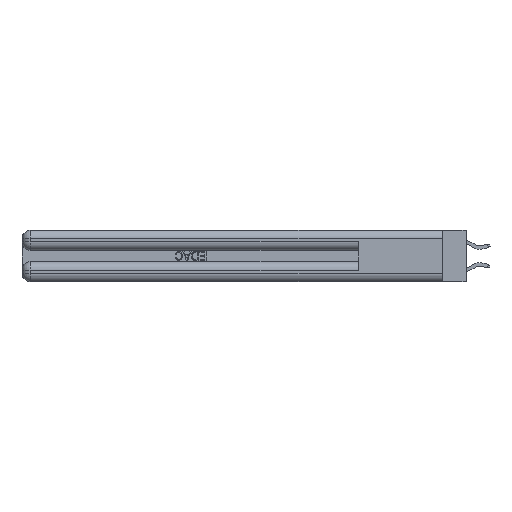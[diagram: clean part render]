
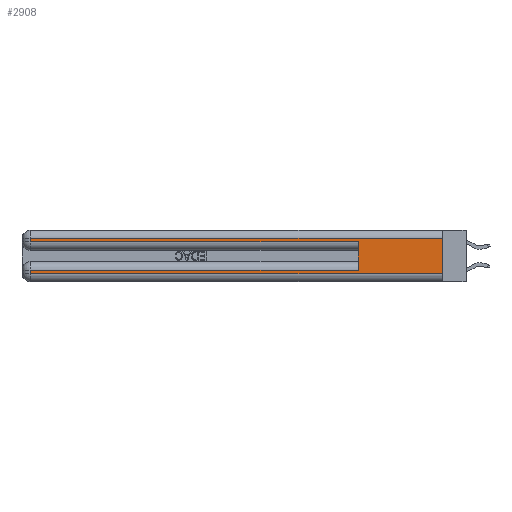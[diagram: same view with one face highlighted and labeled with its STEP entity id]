
A CAD part, left-side view. The second image highlights one B-rep face of the part: STEP entity #2908.
In plain terms, the highlighted planar face has unit normal (-1, 0, 0).
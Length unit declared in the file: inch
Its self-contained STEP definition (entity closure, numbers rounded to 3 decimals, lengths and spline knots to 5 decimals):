
#225 = ORIENTED_EDGE ( 'NONE', *, *, #33813, .T. ) ;
#605 = VERTEX_POINT ( 'NONE', #23759 ) ;
#2132 = EDGE_CURVE ( 'NONE', #27821, #29913, #11934, .T. ) ;
#2157 = VECTOR ( 'NONE', #27868, 39.37008 ) ;
#2297 = VERTEX_POINT ( 'NONE', #30778 ) ;
#2908 = ADVANCED_FACE ( 'NONE', ( #24517 ), #19023, .F. ) ;
#3054 = CARTESIAN_POINT ( 'NONE',  ( 0., 0., 0.37 ) ) ;
#3817 = VERTEX_POINT ( 'NONE', #20271 ) ;
#4042 = VECTOR ( 'NONE', #32883, 39.37008 ) ;
#4208 = EDGE_CURVE ( 'NONE', #2297, #29913, #4775, .T. ) ;
#4294 = LINE ( 'NONE', #22469, #11377 ) ;
#4775 = LINE ( 'NONE', #24913, #25253 ) ;
#4833 = CARTESIAN_POINT ( 'NONE',  ( 0., 2.94, 0.37 ) ) ;
#5351 = DIRECTION ( 'NONE',  ( 0., -1., 0. ) ) ;
#5700 = DIRECTION ( 'NONE',  ( 0., 0., -1. ) ) ;
#5804 = LINE ( 'NONE', #32035, #13721 ) ;
#6391 = CARTESIAN_POINT ( 'NONE',  ( 0., 2.94, 0.285 ) ) ;
#6636 = VERTEX_POINT ( 'NONE', #18787 ) ;
#6854 = CARTESIAN_POINT ( 'NONE',  ( 0., 2.94, 0.085 ) ) ;
#7870 = VECTOR ( 'NONE', #5351, 39.37008 ) ;
#8067 = ORIENTED_EDGE ( 'NONE', *, *, #21373, .T. ) ;
#8251 = CARTESIAN_POINT ( 'NONE',  ( 0., 2.94, 0.37 ) ) ;
#8323 = ORIENTED_EDGE ( 'NONE', *, *, #4208, .F. ) ;
#8755 = ORIENTED_EDGE ( 'NONE', *, *, #17038, .T. ) ;
#9690 = ORIENTED_EDGE ( 'NONE', *, *, #26692, .T. ) ;
#10274 = VERTEX_POINT ( 'NONE', #22075 ) ;
#10942 = DIRECTION ( 'NONE',  ( 0., 0., -1. ) ) ;
#11377 = VECTOR ( 'NONE', #33187, 39.37008 ) ;
#11934 = LINE ( 'NONE', #16774, #4042 ) ;
#13270 = CARTESIAN_POINT ( 'NONE',  ( 0., 0., 0.06 ) ) ;
#13721 = VECTOR ( 'NONE', #24103, 39.37008 ) ;
#14978 = LINE ( 'NONE', #13270, #7870 ) ;
#15521 = ORIENTED_EDGE ( 'NONE', *, *, #23359, .F. ) ;
#16385 = DIRECTION ( 'NONE',  ( 0., 0., 1. ) ) ;
#16407 = LINE ( 'NONE', #4833, #29780 ) ;
#16774 = CARTESIAN_POINT ( 'NONE',  ( 0., 0., 0.285 ) ) ;
#17038 = EDGE_CURVE ( 'NONE', #6636, #3817, #14978, .T. ) ;
#18787 = CARTESIAN_POINT ( 'NONE',  ( 0., 2.94, 0.06 ) ) ;
#19023 = PLANE ( 'NONE',  #24604 ) ;
#19372 = CARTESIAN_POINT ( 'NONE',  ( 0., 0.6, 0.285 ) ) ;
#20271 = CARTESIAN_POINT ( 'NONE',  ( 0., 0., 0.06 ) ) ;
#21373 = EDGE_CURVE ( 'NONE', #605, #27821, #16407, .T. ) ;
#21737 = DIRECTION ( 'NONE',  ( 1., 0., 0. ) ) ;
#22075 = CARTESIAN_POINT ( 'NONE',  ( 0., 0., 0.31 ) ) ;
#22469 = CARTESIAN_POINT ( 'NONE',  ( 0., 0., 0.085 ) ) ;
#23115 = EDGE_LOOP ( 'NONE', ( #15521, #25544, #8067, #25269, #8323, #9690, #225, #8755 ) ) ;
#23359 = EDGE_CURVE ( 'NONE', #10274, #3817, #5804, .T. ) ;
#23451 = LINE ( 'NONE', #25200, #2157 ) ;
#23759 = CARTESIAN_POINT ( 'NONE',  ( 0., 2.94, 0.31 ) ) ;
#23875 = VECTOR ( 'NONE', #10942, 39.37008 ) ;
#24103 = DIRECTION ( 'NONE',  ( 0., 0., -1. ) ) ;
#24517 = FACE_OUTER_BOUND ( 'NONE', #23115, .T. ) ;
#24604 = AXIS2_PLACEMENT_3D ( 'NONE', #3054, #21737, #5700 ) ;
#24721 = LINE ( 'NONE', #8251, #23875 ) ;
#24913 = CARTESIAN_POINT ( 'NONE',  ( 0., 0.6, 0.145 ) ) ;
#25200 = CARTESIAN_POINT ( 'NONE',  ( 0., 0., 0.31 ) ) ;
#25253 = VECTOR ( 'NONE', #16385, 39.37008 ) ;
#25269 = ORIENTED_EDGE ( 'NONE', *, *, #2132, .T. ) ;
#25544 = ORIENTED_EDGE ( 'NONE', *, *, #34051, .T. ) ;
#26692 = EDGE_CURVE ( 'NONE', #2297, #27956, #4294, .T. ) ;
#27821 = VERTEX_POINT ( 'NONE', #6391 ) ;
#27868 = DIRECTION ( 'NONE',  ( 0., 1., 0. ) ) ;
#27956 = VERTEX_POINT ( 'NONE', #6854 ) ;
#29780 = VECTOR ( 'NONE', #34103, 39.37008 ) ;
#29913 = VERTEX_POINT ( 'NONE', #19372 ) ;
#30778 = CARTESIAN_POINT ( 'NONE',  ( 0., 0.6, 0.085 ) ) ;
#32035 = CARTESIAN_POINT ( 'NONE',  ( 0., 0., 0.37 ) ) ;
#32883 = DIRECTION ( 'NONE',  ( 0., -1., 0. ) ) ;
#33187 = DIRECTION ( 'NONE',  ( 0., 1., 0. ) ) ;
#33813 = EDGE_CURVE ( 'NONE', #27956, #6636, #24721, .T. ) ;
#34051 = EDGE_CURVE ( 'NONE', #10274, #605, #23451, .T. ) ;
#34103 = DIRECTION ( 'NONE',  ( 0., 0., -1. ) ) ;
